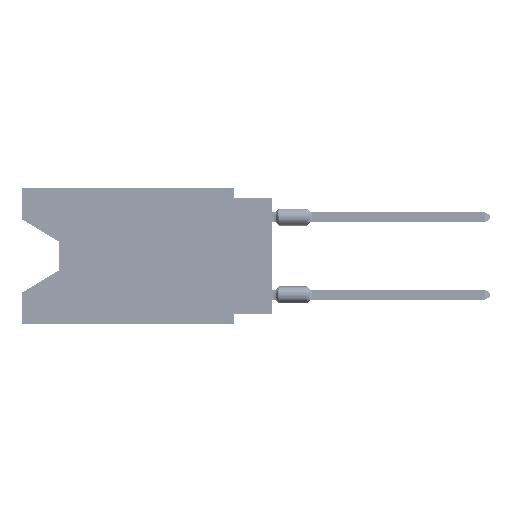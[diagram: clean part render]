
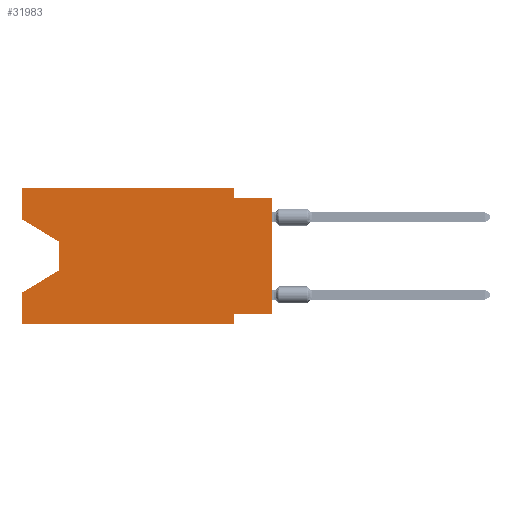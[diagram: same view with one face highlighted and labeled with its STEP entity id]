
A CAD part, left-side view. The second image highlights one B-rep face of the part: STEP entity #31983.
In plain terms, the highlighted planar face has unit normal (-1, 0, 0).
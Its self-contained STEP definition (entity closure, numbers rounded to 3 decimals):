
#94 = VECTOR ( 'NONE', #21058, 1000. ) ;
#1500 = CARTESIAN_POINT ( 'NONE',  ( 0., 13.97, -3.505 ) ) ;
#1580 = LINE ( 'NONE', #75253, #57046 ) ;
#2055 = ORIENTED_EDGE ( 'NONE', *, *, #48081, .F. ) ;
#2230 = EDGE_CURVE ( 'NONE', #19993, #26458, #47952, .T. ) ;
#2360 = ORIENTED_EDGE ( 'NONE', *, *, #25863, .T. ) ;
#2721 = LINE ( 'NONE', #20940, #30575 ) ;
#3239 = DIRECTION ( 'NONE',  ( 0., -1., 0. ) ) ;
#3383 = EDGE_CURVE ( 'NONE', #32623, #42413, #35199, .T. ) ;
#3518 = DIRECTION ( 'NONE',  ( 0., 0., 1. ) ) ;
#5081 = ORIENTED_EDGE ( 'NONE', *, *, #62919, .T. ) ;
#7323 = ORIENTED_EDGE ( 'NONE', *, *, #50896, .F. ) ;
#10633 = DIRECTION ( 'NONE',  ( 0., 0., -1. ) ) ;
#14041 = DIRECTION ( 'NONE',  ( 1., 0., 0. ) ) ;
#14325 = VERTEX_POINT ( 'NONE', #35481 ) ;
#15211 = VECTOR ( 'NONE', #66581, 1000. ) ;
#15823 = CARTESIAN_POINT ( 'NONE',  ( 0., 2.54, 0. ) ) ;
#15887 = LINE ( 'NONE', #34511, #51037 ) ;
#16113 = EDGE_CURVE ( 'NONE', #17496, #59327, #63678, .T. ) ;
#17496 = VERTEX_POINT ( 'NONE', #79045 ) ;
#18286 = ORIENTED_EDGE ( 'NONE', *, *, #47940, .F. ) ;
#18408 = ORIENTED_EDGE ( 'NONE', *, *, #2230, .T. ) ;
#18934 = CARTESIAN_POINT ( 'NONE',  ( 0., 16.383, -8.89 ) ) ;
#19452 = LINE ( 'NONE', #70030, #94 ) ;
#19993 = VERTEX_POINT ( 'NONE', #29542 ) ;
#20853 = LINE ( 'NONE', #44724, #47373 ) ;
#20940 = CARTESIAN_POINT ( 'NONE',  ( 0., 16.383, 0. ) ) ;
#21058 = DIRECTION ( 'NONE',  ( 0., 0., -1. ) ) ;
#21452 = DIRECTION ( 'NONE',  ( 0., 0., 1. ) ) ;
#21502 = ORIENTED_EDGE ( 'NONE', *, *, #16113, .T. ) ;
#21791 = VERTEX_POINT ( 'NONE', #40216 ) ;
#21813 = AXIS2_PLACEMENT_3D ( 'NONE', #63023, #14041, #57342 ) ;
#22919 = EDGE_LOOP ( 'NONE', ( #42870, #2360, #21502, #27027, #5081, #2055, #70782, #18408, #51481, #18286, #7323, #63451 ) ) ;
#25863 = EDGE_CURVE ( 'NONE', #32037, #17496, #15887, .T. ) ;
#26458 = VERTEX_POINT ( 'NONE', #62940 ) ;
#27027 = ORIENTED_EDGE ( 'NONE', *, *, #29896, .F. ) ;
#27519 = CARTESIAN_POINT ( 'NONE',  ( 0., 16.383, 0. ) ) ;
#29542 = CARTESIAN_POINT ( 'NONE',  ( 0., 0., -8.255 ) ) ;
#29896 = EDGE_CURVE ( 'NONE', #71566, #59327, #2721, .T. ) ;
#30002 = DIRECTION ( 'NONE',  ( 0., 0., -1. ) ) ;
#30575 = VECTOR ( 'NONE', #3518, 1000. ) ;
#31492 = LINE ( 'NONE', #48921, #56713 ) ;
#31983 = ADVANCED_FACE ( 'NONE', ( #74374 ), #68693, .F. ) ;
#32037 = VERTEX_POINT ( 'NONE', #1500 ) ;
#32623 = VERTEX_POINT ( 'NONE', #36449 ) ;
#33325 = EDGE_CURVE ( 'NONE', #78135, #26458, #53198, .T. ) ;
#34511 = CARTESIAN_POINT ( 'NONE',  ( 0., 13.97, -3.505 ) ) ;
#35199 = LINE ( 'NONE', #27519, #46336 ) ;
#35481 = CARTESIAN_POINT ( 'NONE',  ( 0., 2.54, -8.89 ) ) ;
#36073 = LINE ( 'NONE', #49399, #53020 ) ;
#36289 = CARTESIAN_POINT ( 'NONE',  ( 0., 16.383, 0. ) ) ;
#36449 = CARTESIAN_POINT ( 'NONE',  ( 0., 16.383, -2.038 ) ) ;
#40216 = CARTESIAN_POINT ( 'NONE',  ( 0., 2.54, -8.255 ) ) ;
#42413 = VERTEX_POINT ( 'NONE', #36289 ) ;
#42870 = ORIENTED_EDGE ( 'NONE', *, *, #63232, .T. ) ;
#44326 = DIRECTION ( 'NONE',  ( 0., 1., 0. ) ) ;
#44470 = DIRECTION ( 'NONE',  ( 0., -1., 0. ) ) ;
#44724 = CARTESIAN_POINT ( 'NONE',  ( 0., 0., -8.255 ) ) ;
#44795 = VERTEX_POINT ( 'NONE', #15823 ) ;
#45592 = VECTOR ( 'NONE', #68960, 1000. ) ;
#46336 = VECTOR ( 'NONE', #21452, 1000. ) ;
#47118 = DIRECTION ( 'NONE',  ( 0., -1., 0. ) ) ;
#47373 = VECTOR ( 'NONE', #44326, 1000. ) ;
#47940 = EDGE_CURVE ( 'NONE', #44795, #78135, #36073, .T. ) ;
#47952 = LINE ( 'NONE', #72659, #15211 ) ;
#48081 = EDGE_CURVE ( 'NONE', #21791, #14325, #19452, .T. ) ;
#48921 = CARTESIAN_POINT ( 'NONE',  ( 0., 16.383, -2.038 ) ) ;
#49399 = CARTESIAN_POINT ( 'NONE',  ( 0., 2.54, 0. ) ) ;
#50314 = VECTOR ( 'NONE', #47118, 1000. ) ;
#50896 = EDGE_CURVE ( 'NONE', #42413, #44795, #1580, .T. ) ;
#51037 = VECTOR ( 'NONE', #10633, 1000. ) ;
#51481 = ORIENTED_EDGE ( 'NONE', *, *, #33325, .F. ) ;
#53020 = VECTOR ( 'NONE', #30002, 1000. ) ;
#53198 = LINE ( 'NONE', #77890, #50314 ) ;
#56175 = DIRECTION ( 'NONE',  ( 0., -0.855, -0.519 ) ) ;
#56713 = VECTOR ( 'NONE', #56175, 1000. ) ;
#57046 = VECTOR ( 'NONE', #44470, 1000. ) ;
#57205 = CARTESIAN_POINT ( 'NONE',  ( 0., 13.97, -5.385 ) ) ;
#57342 = DIRECTION ( 'NONE',  ( 0., 0., -1. ) ) ;
#59327 = VERTEX_POINT ( 'NONE', #66764 ) ;
#62919 = EDGE_CURVE ( 'NONE', #71566, #14325, #71252, .T. ) ;
#62940 = CARTESIAN_POINT ( 'NONE',  ( 0., 0., -0.635 ) ) ;
#63023 = CARTESIAN_POINT ( 'NONE',  ( 0., 16.383, 0. ) ) ;
#63232 = EDGE_CURVE ( 'NONE', #32623, #32037, #31492, .T. ) ;
#63451 = ORIENTED_EDGE ( 'NONE', *, *, #3383, .F. ) ;
#63678 = LINE ( 'NONE', #57205, #45592 ) ;
#64362 = CARTESIAN_POINT ( 'NONE',  ( 0., 16.383, -8.89 ) ) ;
#64538 = VECTOR ( 'NONE', #3239, 1000. ) ;
#66581 = DIRECTION ( 'NONE',  ( 0., 0., 1. ) ) ;
#66764 = CARTESIAN_POINT ( 'NONE',  ( 0., 16.383, -6.852 ) ) ;
#68693 = PLANE ( 'NONE',  #21813 ) ;
#68960 = DIRECTION ( 'NONE',  ( 0., 0.855, -0.519 ) ) ;
#70030 = CARTESIAN_POINT ( 'NONE',  ( 0., 2.54, -8.89 ) ) ;
#70782 = ORIENTED_EDGE ( 'NONE', *, *, #73385, .F. ) ;
#71252 = LINE ( 'NONE', #64362, #64538 ) ;
#71566 = VERTEX_POINT ( 'NONE', #18934 ) ;
#72598 = CARTESIAN_POINT ( 'NONE',  ( 0., 2.54, -0.635 ) ) ;
#72659 = CARTESIAN_POINT ( 'NONE',  ( 0., 0., 0. ) ) ;
#73385 = EDGE_CURVE ( 'NONE', #19993, #21791, #20853, .T. ) ;
#74374 = FACE_OUTER_BOUND ( 'NONE', #22919, .T. ) ;
#75253 = CARTESIAN_POINT ( 'NONE',  ( 0., 16.383, 0. ) ) ;
#77890 = CARTESIAN_POINT ( 'NONE',  ( 0., 0., -0.635 ) ) ;
#78135 = VERTEX_POINT ( 'NONE', #72598 ) ;
#79045 = CARTESIAN_POINT ( 'NONE',  ( 0., 13.97, -5.385 ) ) ;
